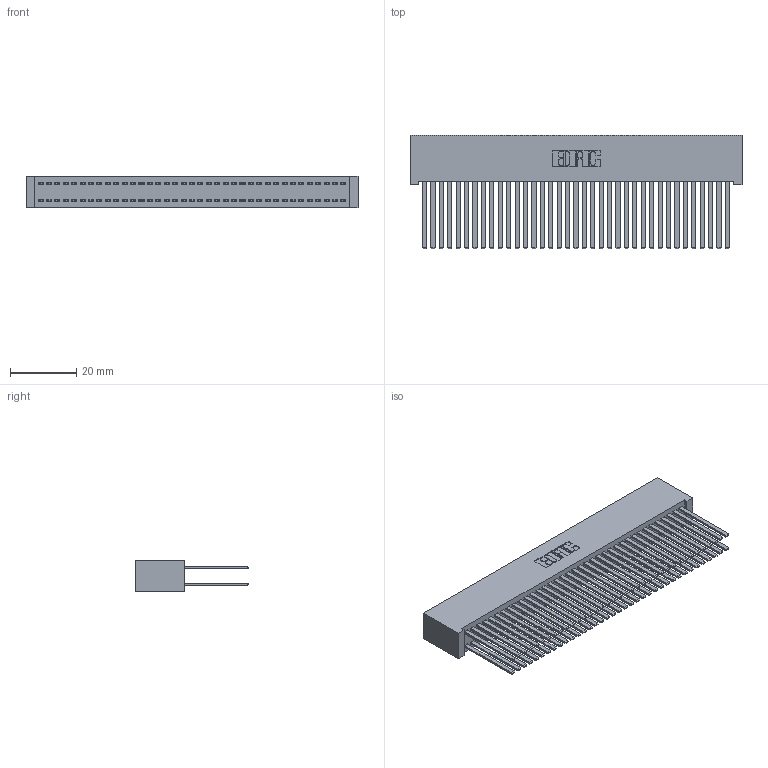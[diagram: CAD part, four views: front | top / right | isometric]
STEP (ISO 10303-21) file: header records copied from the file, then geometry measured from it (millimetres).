
FILE_DESCRIPTION (( 'STEP AP203' ), '1' );
FILE_NAME ('342-074-544-201.STEP', '2019-10-03T17:19:47', ( '' ), ( '' ), 'SwSTEP 2.0', 'SolidWorks 2016', '' );
FILE_SCHEMA (( 'CONFIG_CONTROL_DESIGN' ));
Length unit declared in the file: inch
Products named in the file (3): 345-292-001_345-293-144; 342-074-544-201; 342 Part_Lugless
Assembly tree (75 placements, depth 2):
  342-074-544-201
    342 Part_Lugless
    345-292-001_345-293-144  x74
Bounding box: 100.23 x 34.3 x 9.4 mm (x, y, z)
Volume: 10458.7 mm3; surface area: 20219.9 mm2
Topology: 75 solids, 75 shells, 3506 faces, 10413 edges, 6842 vertices
Faces by surface type: plane 2430, cylinder 1076
Entity records: 23857 total; most frequent: CARTESIAN_POINT 3954, ORIENTED_EDGE 3890, DIRECTION 3377, EDGE_CURVE 1945, VECTOR 1829, LINE 1829, VERTEX_POINT 1294, AXIS2_PLACEMENT_3D 774
